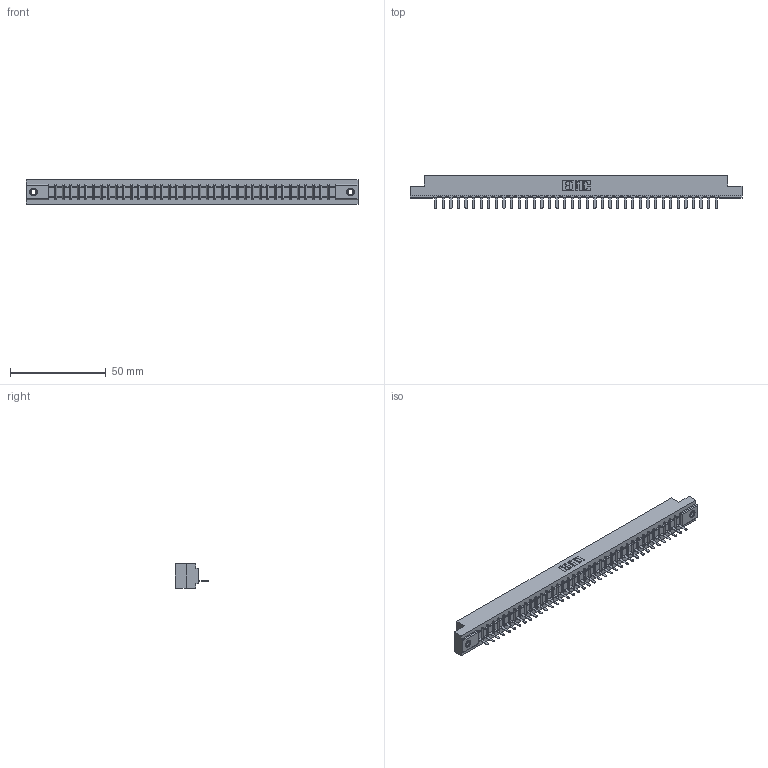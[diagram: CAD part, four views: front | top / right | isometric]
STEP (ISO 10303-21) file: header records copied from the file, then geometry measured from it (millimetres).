
FILE_DESCRIPTION (( 'STEP AP203' ), '1' );
FILE_NAME ('307-038-521-107.STEP', '2018-08-05T11:09:19', ( '' ), ( '' ), 'SwSTEP 2.0', 'SolidWorks 2016', '' );
FILE_SCHEMA (( 'CONFIG_CONTROL_DESIGN' ));
Length unit declared in the file: inch
Products named in the file (4): 307 Part_.156 Dia Mounting Holes; 307-290-002_521; 345-250-001_345-250-005-103; 307-038-521-107
Assembly tree (41 placements, depth 2):
  307-038-521-107
    307 Part_.156 Dia Mounting Holes
    307-290-002_521  x38
    345-250-001_345-250-005-103  x2
Bounding box: 173.58 x 17.42 x 12.7 mm (x, y, z)
Volume: 18534.5 mm3; surface area: 23255.8 mm2
Topology: 41 solids, 41 shells, 3029 faces, 9275 edges, 6070 vertices
Faces by surface type: plane 1812, cylinder 1123, sphere 78, cone 12, torus 4
Entity records: 34973 total; most frequent: CARTESIAN_POINT 5879, ORIENTED_EDGE 5862, DIRECTION 5723, EDGE_CURVE 2931, LINE 2243, VECTOR 2243, VERTEX_POINT 1896, AXIS2_PLACEMENT_3D 1740
